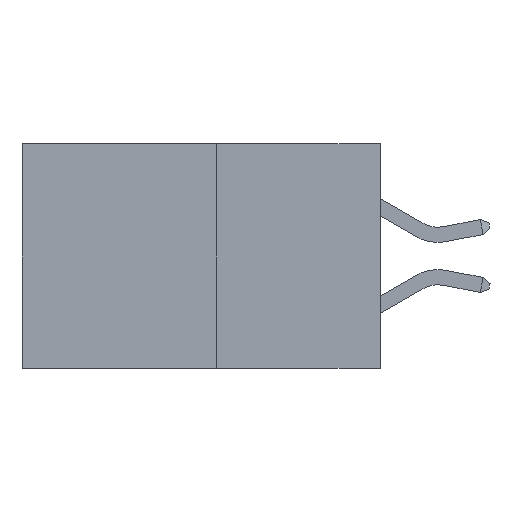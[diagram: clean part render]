
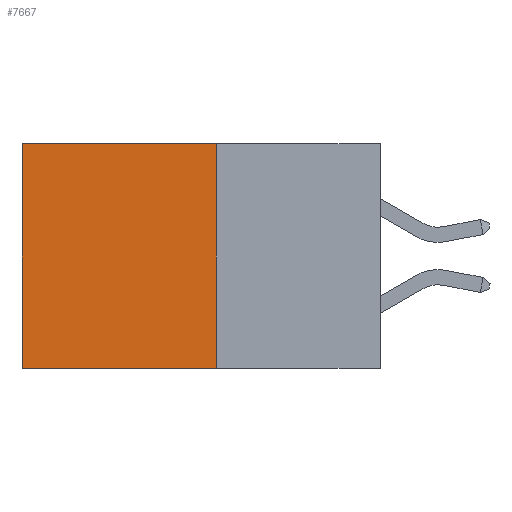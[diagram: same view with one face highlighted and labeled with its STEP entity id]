
A CAD part, left-side view. The second image highlights one B-rep face of the part: STEP entity #7667.
In plain terms, the highlighted planar face has unit normal (-1, 0, 0).
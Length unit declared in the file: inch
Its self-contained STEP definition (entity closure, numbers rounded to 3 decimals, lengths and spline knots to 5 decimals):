
#90 = VERTEX_POINT ( 'NONE', #20829 ) ;
#312 = VERTEX_POINT ( 'NONE', #9122 ) ;
#316 = ORIENTED_EDGE ( 'NONE', *, *, #485, .T. ) ;
#485 = EDGE_CURVE ( 'NONE', #19551, #21732, #2919, .T. ) ;
#977 = DIRECTION ( 'NONE',  ( 0., 0., -1. ) ) ;
#2383 = VECTOR ( 'NONE', #21865, 39.37008 ) ;
#2919 = LINE ( 'NONE', #18683, #2383 ) ;
#2994 = DIRECTION ( 'NONE',  ( 0., 0., -1. ) ) ;
#3404 = CARTESIAN_POINT ( 'NONE',  ( 0.277, 0.59, 0. ) ) ;
#3410 = CARTESIAN_POINT ( 'NONE',  ( 0.277, 0.27, -0.37 ) ) ;
#4039 = FACE_OUTER_BOUND ( 'NONE', #12475, .T. ) ;
#6033 = EDGE_CURVE ( 'NONE', #21732, #312, #18609, .T. ) ;
#7667 = ADVANCED_FACE ( 'NONE', ( #4039 ), #18098, .F. ) ;
#7716 = EDGE_CURVE ( 'NONE', #90, #312, #12119, .T. ) ;
#9122 = CARTESIAN_POINT ( 'NONE',  ( 0.277, 0.59, -0.37 ) ) ;
#9780 = AXIS2_PLACEMENT_3D ( 'NONE', #21478, #11297, #977 ) ;
#11297 = DIRECTION ( 'NONE',  ( 1., 0., 0. ) ) ;
#11576 = VECTOR ( 'NONE', #16528, 39.37008 ) ;
#11871 = CARTESIAN_POINT ( 'NONE',  ( 0.277, 0.27, 0. ) ) ;
#12119 = LINE ( 'NONE', #21548, #11576 ) ;
#12125 = ORIENTED_EDGE ( 'NONE', *, *, #18898, .F. ) ;
#12475 = EDGE_LOOP ( 'NONE', ( #16129, #19332, #12125, #316 ) ) ;
#14060 = VECTOR ( 'NONE', #2994, 39.37008 ) ;
#14567 = VECTOR ( 'NONE', #17152, 39.37008 ) ;
#16129 = ORIENTED_EDGE ( 'NONE', *, *, #6033, .T. ) ;
#16528 = DIRECTION ( 'NONE',  ( 0., 1., 0. ) ) ;
#17152 = DIRECTION ( 'NONE',  ( 0., 0., -1. ) ) ;
#18098 = PLANE ( 'NONE',  #9780 ) ;
#18581 = LINE ( 'NONE', #3410, #14567 ) ;
#18609 = LINE ( 'NONE', #21767, #14060 ) ;
#18683 = CARTESIAN_POINT ( 'NONE',  ( 0.277, 0.27, 0. ) ) ;
#18898 = EDGE_CURVE ( 'NONE', #19551, #90, #18581, .T. ) ;
#19332 = ORIENTED_EDGE ( 'NONE', *, *, #7716, .F. ) ;
#19551 = VERTEX_POINT ( 'NONE', #11871 ) ;
#20829 = CARTESIAN_POINT ( 'NONE',  ( 0.277, 0.27, -0.37 ) ) ;
#21478 = CARTESIAN_POINT ( 'NONE',  ( 0.277, 0.27, -0.37 ) ) ;
#21548 = CARTESIAN_POINT ( 'NONE',  ( 0.277, 0.27, -0.37 ) ) ;
#21732 = VERTEX_POINT ( 'NONE', #3404 ) ;
#21767 = CARTESIAN_POINT ( 'NONE',  ( 0.277, 0.59, -0.37 ) ) ;
#21865 = DIRECTION ( 'NONE',  ( 0., 1., 0. ) ) ;
